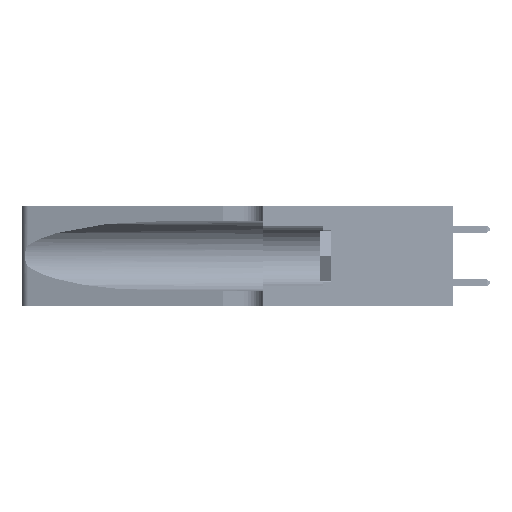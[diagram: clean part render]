
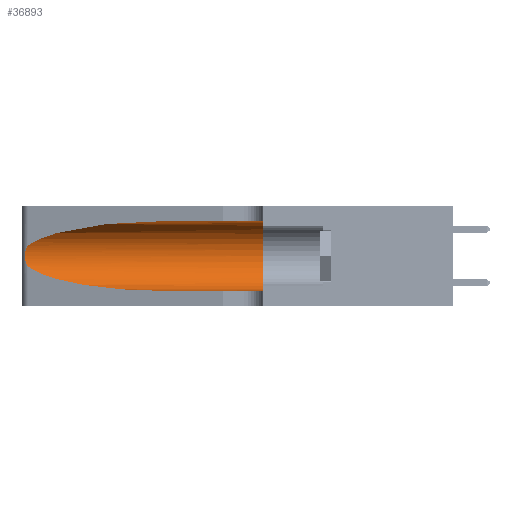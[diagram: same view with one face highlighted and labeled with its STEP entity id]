
A CAD part, left-side view. The second image highlights one B-rep face of the part: STEP entity #36893.
In plain terms, the highlighted cylindrical face has radius 3.308 mm (diameter 6.617 mm), a partial arc.
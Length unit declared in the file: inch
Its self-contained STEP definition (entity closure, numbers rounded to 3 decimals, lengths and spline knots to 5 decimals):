
#634 = LINE ( 'NONE', #4420, #14181 ) ;
#726 = CYLINDRICAL_SURFACE ( 'NONE', #18074, 0.13025 ) ;
#1047 = CIRCLE ( 'NONE', #15203, 0.13025 ) ;
#1191 = CARTESIAN_POINT ( 'NONE',  ( 0.26075, 1.23896, 0.19203 ) ) ;
#4349 = CARTESIAN_POINT ( 'NONE',  ( 0.18966, 0.96281, 0.31525 ) ) ;
#4420 = CARTESIAN_POINT ( 'NONE',  ( 0.1305, 1.61858, 0.05475 ) ) ;
#4932 = CARTESIAN_POINT ( 'NONE',  ( 0.25487, 1.22718, 0.14631 ) ) ;
#5314 = CARTESIAN_POINT ( 'NONE',  ( 0.25854, 1.2359, 0.20912 ) ) ;
#7847 =( BOUNDED_CURVE ( )  B_SPLINE_CURVE ( 3, ( #4932, #32407, #28460, #36335 ),
 .UNSPECIFIED., .F., .F. ) 
 B_SPLINE_CURVE_WITH_KNOTS ( ( 4, 4 ),
 ( 3.44316, 4.71239 ),
 .UNSPECIFIED. ) 
 CURVE ( )  GEOMETRIC_REPRESENTATION_ITEM ( )  RATIONAL_B_SPLINE_CURVE ( ( 1., 0.87, 0.87, 1. ) ) 
 REPRESENTATION_ITEM ( '' )  );
#8097 = DIRECTION ( 'NONE',  ( 0., 0., -1. ) ) ;
#10632 = FACE_OUTER_BOUND ( 'NONE', #25836, .T. ) ;
#12454 = VERTEX_POINT ( 'NONE', #37234 ) ;
#12917 = CARTESIAN_POINT ( 'NONE',  ( 0.25789, 1.23486, 0.15765 ) ) ;
#13053 = LINE ( 'NONE', #37530, #45553 ) ;
#13212 = DIRECTION ( 'NONE',  ( 0., -1., 0. ) ) ;
#14181 = VECTOR ( 'NONE', #13212, 39.37008 ) ;
#15203 = AXIS2_PLACEMENT_3D ( 'NONE', #35238, #25828, #35923 ) ;
#15568 = CARTESIAN_POINT ( 'NONE',  ( 0.2373, 1.15595, 0.28018 ) ) ;
#16890 = CARTESIAN_POINT ( 'NONE',  ( 0.25555, 1.22994, 0.2215 ) ) ;
#17052 = CARTESIAN_POINT ( 'NONE',  ( 0.25856, 1.23593, 0.16098 ) ) ;
#18074 = AXIS2_PLACEMENT_3D ( 'NONE', #26995, #42939, #8097 ) ;
#18559 = VERTEX_POINT ( 'NONE', #42190 ) ;
#19106 = ORIENTED_EDGE ( 'NONE', *, *, #50667, .F. ) ;
#20124 = EDGE_CURVE ( 'NONE', #37697, #32034, #7847, .T. ) ;
#20621 = CARTESIAN_POINT ( 'NONE',  ( 0.26075, 1.23896, 0.178 ) ) ;
#20964 = CARTESIAN_POINT ( 'NONE',  ( 0.25487, 1.22718, 0.14631 ) ) ;
#23747 = CARTESIAN_POINT ( 'NONE',  ( 0.25487, 1.22718, 0.22369 ) ) ;
#24368 = CARTESIAN_POINT ( 'NONE',  ( 0.26017, 1.23833, 0.17102 ) ) ;
#25828 = DIRECTION ( 'NONE',  ( 0., 1., 0. ) ) ;
#25836 = EDGE_LOOP ( 'NONE', ( #50377, #36940, #49699, #50552, #34685, #19106 ) ) ;
#26995 = CARTESIAN_POINT ( 'NONE',  ( 0.1305, 1.61858, 0.185 ) ) ;
#28460 = CARTESIAN_POINT ( 'NONE',  ( 0.18966, 0.96281, 0.05475 ) ) ;
#32034 = VERTEX_POINT ( 'NONE', #41925 ) ;
#32071 = VERTEX_POINT ( 'NONE', #50006 ) ;
#32407 = CARTESIAN_POINT ( 'NONE',  ( 0.2373, 1.15595, 0.08982 ) ) ;
#32444 = CARTESIAN_POINT ( 'NONE',  ( 0.25487, 1.22718, 0.22369 ) ) ;
#32622 = CARTESIAN_POINT ( 'NONE',  ( 0.26018, 1.23835, 0.19895 ) ) ;
#33559 = CARTESIAN_POINT ( 'NONE',  ( 0.1305, 0.72297, 0.31525 ) ) ;
#34685 = ORIENTED_EDGE ( 'NONE', *, *, #40470, .F. ) ;
#35238 = CARTESIAN_POINT ( 'NONE',  ( 0.1305, 0.35, 0.185 ) ) ;
#35923 = DIRECTION ( 'NONE',  ( 0., 0., 1. ) ) ;
#36144 = CARTESIAN_POINT ( 'NONE',  ( 0.25487, 1.22718, 0.14631 ) ) ;
#36335 = CARTESIAN_POINT ( 'NONE',  ( 0.1305, 0.72297, 0.05475 ) ) ;
#36790 = B_SPLINE_CURVE_WITH_KNOTS ( 'NONE', 3,
 ( #32444, #16890, #47898, #40518, #5314, #32622, #1191, #20621, #24368, #17052, #12917, #44271, #48082, #20964 ),
 .UNSPECIFIED., .F., .F.,
 ( 4, 2, 2, 2, 2, 2, 4 ),
 ( 0., 0.00027, 0.00053, 0.00107, 0.0016, 0.00187, 0.00214 ),
 .UNSPECIFIED. ) ;
#36893 = ADVANCED_FACE ( 'NONE', ( #10632 ), #726, .F. ) ;
#36940 = ORIENTED_EDGE ( 'NONE', *, *, #37072, .T. ) ;
#37072 = EDGE_CURVE ( 'NONE', #18559, #37697, #36790, .T. ) ;
#37234 = CARTESIAN_POINT ( 'NONE',  ( 0.1305, 0.35, 0.05475 ) ) ;
#37530 = CARTESIAN_POINT ( 'NONE',  ( 0.1305, 1.61858, 0.31525 ) ) ;
#37697 = VERTEX_POINT ( 'NONE', #36144 ) ;
#39001 =( BOUNDED_CURVE ( )  B_SPLINE_CURVE ( 3, ( #47278, #4349, #15568, #23747 ),
 .UNSPECIFIED., .F., .F. ) 
 B_SPLINE_CURVE_WITH_KNOTS ( ( 4, 4 ),
 ( 1.5708, 2.84003 ),
 .UNSPECIFIED. ) 
 CURVE ( )  GEOMETRIC_REPRESENTATION_ITEM ( )  RATIONAL_B_SPLINE_CURVE ( ( 1., 0.87, 0.87, 1. ) ) 
 REPRESENTATION_ITEM ( '' )  );
#40470 = EDGE_CURVE ( 'NONE', #32071, #12454, #1047, .T. ) ;
#40518 = CARTESIAN_POINT ( 'NONE',  ( 0.25787, 1.23484, 0.2124 ) ) ;
#41925 = CARTESIAN_POINT ( 'NONE',  ( 0.1305, 0.72297, 0.05475 ) ) ;
#42190 = CARTESIAN_POINT ( 'NONE',  ( 0.25487, 1.22718, 0.22369 ) ) ;
#42939 = DIRECTION ( 'NONE',  ( 0., -1., 0. ) ) ;
#44271 = CARTESIAN_POINT ( 'NONE',  ( 0.25639, 1.23186, 0.15144 ) ) ;
#44492 = VERTEX_POINT ( 'NONE', #33559 ) ;
#44820 = EDGE_CURVE ( 'NONE', #44492, #18559, #39001, .T. ) ;
#45553 = VECTOR ( 'NONE', #49397, 39.37008 ) ;
#46242 = EDGE_CURVE ( 'NONE', #32034, #12454, #634, .T. ) ;
#47278 = CARTESIAN_POINT ( 'NONE',  ( 0.1305, 0.72297, 0.31525 ) ) ;
#47898 = CARTESIAN_POINT ( 'NONE',  ( 0.25639, 1.23184, 0.21858 ) ) ;
#48082 = CARTESIAN_POINT ( 'NONE',  ( 0.25555, 1.22993, 0.14849 ) ) ;
#49397 = DIRECTION ( 'NONE',  ( 0., -1., 0. ) ) ;
#49699 = ORIENTED_EDGE ( 'NONE', *, *, #20124, .T. ) ;
#50006 = CARTESIAN_POINT ( 'NONE',  ( 0.1305, 0.35, 0.31525 ) ) ;
#50377 = ORIENTED_EDGE ( 'NONE', *, *, #44820, .T. ) ;
#50552 = ORIENTED_EDGE ( 'NONE', *, *, #46242, .T. ) ;
#50667 = EDGE_CURVE ( 'NONE', #44492, #32071, #13053, .T. ) ;
